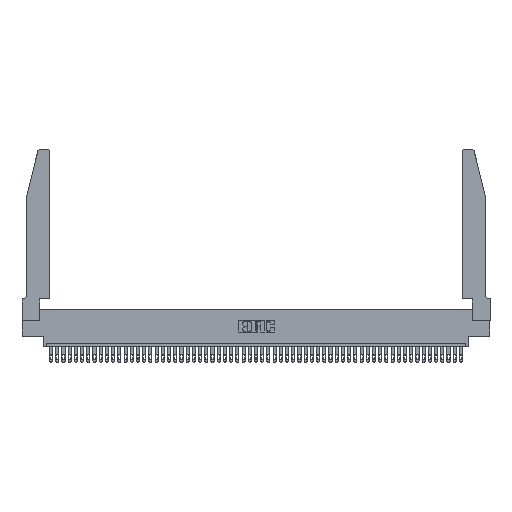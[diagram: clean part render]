
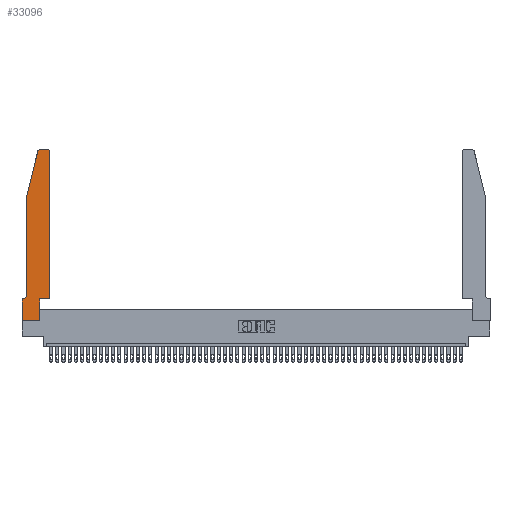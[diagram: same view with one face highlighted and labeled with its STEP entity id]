
A CAD part, top view. The second image highlights one B-rep face of the part: STEP entity #33096.
In plain terms, the highlighted planar face has unit normal (0, 0, 1).
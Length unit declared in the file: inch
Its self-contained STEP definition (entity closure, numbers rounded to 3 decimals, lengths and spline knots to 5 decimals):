
#367 = ORIENTED_EDGE ( 'NONE', *, *, #51072, .T. ) ;
#444 = CARTESIAN_POINT ( 'NONE',  ( 0.2865, 0.35, 0.37 ) ) ;
#504 = AXIS2_PLACEMENT_3D ( 'NONE', #26801, #51103, #47247 ) ;
#686 = VERTEX_POINT ( 'NONE', #15358 ) ;
#928 = VERTEX_POINT ( 'NONE', #2492 ) ;
#2492 = CARTESIAN_POINT ( 'NONE',  ( 0.2865, 0., 0.37 ) ) ;
#2516 = CARTESIAN_POINT ( 'NONE',  ( 0., 0., 0.37 ) ) ;
#3729 = VECTOR ( 'NONE', #17673, 39.37008 ) ;
#4258 = FACE_OUTER_BOUND ( 'NONE', #47462, .T. ) ;
#5263 = DIRECTION ( 'NONE',  ( 0., 0., -1. ) ) ;
#5512 = EDGE_CURVE ( 'NONE', #686, #23134, #22981, .T. ) ;
#5586 = DIRECTION ( 'NONE',  ( 0., 1., 0. ) ) ;
#6033 = LINE ( 'NONE', #25828, #10372 ) ;
#6786 = ORIENTED_EDGE ( 'NONE', *, *, #5512, .T. ) ;
#7185 = VERTEX_POINT ( 'NONE', #50061 ) ;
#7594 = CARTESIAN_POINT ( 'NONE',  ( 0.4505, 0.35, 0.37 ) ) ;
#9978 = DIRECTION ( 'NONE',  ( -1., 0., 0. ) ) ;
#10372 = VECTOR ( 'NONE', #9978, 39.37008 ) ;
#10462 = DIRECTION ( 'NONE',  ( 0., 0., 1. ) ) ;
#11126 = LINE ( 'NONE', #7594, #38033 ) ;
#11177 = VECTOR ( 'NONE', #16803, 39.37008 ) ;
#13188 = CARTESIAN_POINT ( 'NONE',  ( 0.4505, 0.35, 0.37 ) ) ;
#13649 = CIRCLE ( 'NONE', #47724, 0.07 ) ;
#14054 = ORIENTED_EDGE ( 'NONE', *, *, #44420, .T. ) ;
#14263 = LINE ( 'NONE', #21333, #3729 ) ;
#15027 = LINE ( 'NONE', #21026, #36984 ) ;
#15358 = CARTESIAN_POINT ( 'NONE',  ( 0.0755, 2., 0.37 ) ) ;
#15961 = EDGE_CURVE ( 'NONE', #39104, #928, #14263, .T. ) ;
#16764 = VERTEX_POINT ( 'NONE', #50680 ) ;
#16803 = DIRECTION ( 'NONE',  ( -1., 0., 0. ) ) ;
#16893 = CARTESIAN_POINT ( 'NONE',  ( 0.0055, 0.42, 0.37 ) ) ;
#17243 = EDGE_CURVE ( 'NONE', #16764, #48913, #6033, .T. ) ;
#17630 = LINE ( 'NONE', #2516, #31463 ) ;
#17673 = DIRECTION ( 'NONE',  ( 1., 0., 0. ) ) ;
#17877 = DIRECTION ( 'NONE',  ( 1., 0., 0. ) ) ;
#18112 = LINE ( 'NONE', #38234, #40771 ) ;
#18205 = AXIS2_PLACEMENT_3D ( 'NONE', #26909, #31478, #19178 ) ;
#19124 = ORIENTED_EDGE ( 'NONE', *, *, #15961, .T. ) ;
#19178 = DIRECTION ( 'NONE',  ( 1., 0., 0. ) ) ;
#20088 = VERTEX_POINT ( 'NONE', #40871 ) ;
#20924 = VERTEX_POINT ( 'NONE', #27979 ) ;
#21026 = CARTESIAN_POINT ( 'NONE',  ( 0.4505, 0.35, 0.37 ) ) ;
#21120 = EDGE_CURVE ( 'NONE', #20088, #7185, #31749, .T. ) ;
#21333 = CARTESIAN_POINT ( 'NONE',  ( 0., 0., 0.37 ) ) ;
#22981 = LINE ( 'NONE', #43992, #25423 ) ;
#23134 = VERTEX_POINT ( 'NONE', #31113 ) ;
#23658 = VERTEX_POINT ( 'NONE', #37667 ) ;
#24154 = DIRECTION ( 'NONE',  ( 0., 1., 0. ) ) ;
#24231 = EDGE_CURVE ( 'NONE', #48913, #39104, #17630, .T. ) ;
#24765 = ORIENTED_EDGE ( 'NONE', *, *, #39795, .T. ) ;
#25081 = DIRECTION ( 'NONE',  ( -1., 0., 0. ) ) ;
#25423 = VECTOR ( 'NONE', #27396, 39.37008 ) ;
#25828 = CARTESIAN_POINT ( 'NONE',  ( 0.0755, 0.35, 0.37 ) ) ;
#25967 = EDGE_CURVE ( 'NONE', #7185, #686, #18112, .T. ) ;
#25991 = DIRECTION ( 'NONE',  ( 0., -1., 0. ) ) ;
#26778 = LINE ( 'NONE', #32929, #11177 ) ;
#26801 = CARTESIAN_POINT ( 'NONE',  ( 0.284, 2.72, 0.37 ) ) ;
#26814 = VERTEX_POINT ( 'NONE', #444 ) ;
#26909 = CARTESIAN_POINT ( 'NONE',  ( 0.4205, 2.72, 0.37 ) ) ;
#26993 = ORIENTED_EDGE ( 'NONE', *, *, #27467, .T. ) ;
#27396 = DIRECTION ( 'NONE',  ( 0., -1., 0. ) ) ;
#27467 = EDGE_CURVE ( 'NONE', #23658, #20088, #26778, .T. ) ;
#27639 = EDGE_CURVE ( 'NONE', #26814, #42608, #11126, .T. ) ;
#27976 = ORIENTED_EDGE ( 'NONE', *, *, #21120, .T. ) ;
#27979 = CARTESIAN_POINT ( 'NONE',  ( 0.4505, 2.72, 0.37 ) ) ;
#28220 = CARTESIAN_POINT ( 'NONE',  ( 0.2865, 0.35, 0.37 ) ) ;
#28245 = CARTESIAN_POINT ( 'NONE',  ( 0., 0.35, 0.37 ) ) ;
#29331 = CIRCLE ( 'NONE', #18205, 0.03 ) ;
#29579 = LINE ( 'NONE', #28220, #40361 ) ;
#30173 = ORIENTED_EDGE ( 'NONE', *, *, #27639, .T. ) ;
#31113 = CARTESIAN_POINT ( 'NONE',  ( 0.0755, 0.42, 0.37 ) ) ;
#31463 = VECTOR ( 'NONE', #25991, 39.37008 ) ;
#31478 = DIRECTION ( 'NONE',  ( 0., 0., 1. ) ) ;
#31678 = CARTESIAN_POINT ( 'NONE',  ( 0., 0., 0.37 ) ) ;
#31749 = CIRCLE ( 'NONE', #504, 0.03 ) ;
#32929 = CARTESIAN_POINT ( 'NONE',  ( 0.2605, 2.75, 0.37 ) ) ;
#33096 = ADVANCED_FACE ( 'NONE', ( #4258 ), #34397, .T. ) ;
#34397 = PLANE ( 'NONE',  #49228 ) ;
#36338 = ORIENTED_EDGE ( 'NONE', *, *, #46787, .T. ) ;
#36984 = VECTOR ( 'NONE', #5586, 39.37008 ) ;
#37667 = CARTESIAN_POINT ( 'NONE',  ( 0.4205, 2.75, 0.37 ) ) ;
#38033 = VECTOR ( 'NONE', #50646, 39.37008 ) ;
#38234 = CARTESIAN_POINT ( 'NONE',  ( 0.0755, 2., 0.37 ) ) ;
#39104 = VERTEX_POINT ( 'NONE', #31678 ) ;
#39795 = EDGE_CURVE ( 'NONE', #928, #26814, #29579, .T. ) ;
#40361 = VECTOR ( 'NONE', #24154, 39.37008 ) ;
#40771 = VECTOR ( 'NONE', #46508, 39.37008 ) ;
#40871 = CARTESIAN_POINT ( 'NONE',  ( 0.284, 2.75, 0.37 ) ) ;
#41501 = ORIENTED_EDGE ( 'NONE', *, *, #24231, .T. ) ;
#42608 = VERTEX_POINT ( 'NONE', #13188 ) ;
#43992 = CARTESIAN_POINT ( 'NONE',  ( 0.0755, 2., 0.37 ) ) ;
#44420 = EDGE_CURVE ( 'NONE', #20924, #23658, #29331, .T. ) ;
#46508 = DIRECTION ( 'NONE',  ( -0.239, -0.971, 0. ) ) ;
#46579 = CARTESIAN_POINT ( 'NONE',  ( 0., 0.35, 0.37 ) ) ;
#46787 = EDGE_CURVE ( 'NONE', #42608, #20924, #15027, .T. ) ;
#46849 = ORIENTED_EDGE ( 'NONE', *, *, #25967, .T. ) ;
#47247 = DIRECTION ( 'NONE',  ( 1., 0., 0. ) ) ;
#47462 = EDGE_LOOP ( 'NONE', ( #26993, #27976, #46849, #6786, #367, #49679, #41501, #19124, #24765, #30173, #36338, #14054 ) ) ;
#47724 = AXIS2_PLACEMENT_3D ( 'NONE', #16893, #5263, #25081 ) ;
#48913 = VERTEX_POINT ( 'NONE', #28245 ) ;
#49228 = AXIS2_PLACEMENT_3D ( 'NONE', #46579, #10462, #17877 ) ;
#49679 = ORIENTED_EDGE ( 'NONE', *, *, #17243, .T. ) ;
#50061 = CARTESIAN_POINT ( 'NONE',  ( 0.25487, 2.72718, 0.37 ) ) ;
#50646 = DIRECTION ( 'NONE',  ( 1., 0., 0. ) ) ;
#50680 = CARTESIAN_POINT ( 'NONE',  ( 0.0055, 0.35, 0.37 ) ) ;
#51072 = EDGE_CURVE ( 'NONE', #23134, #16764, #13649, .T. ) ;
#51103 = DIRECTION ( 'NONE',  ( 0., 0., 1. ) ) ;
